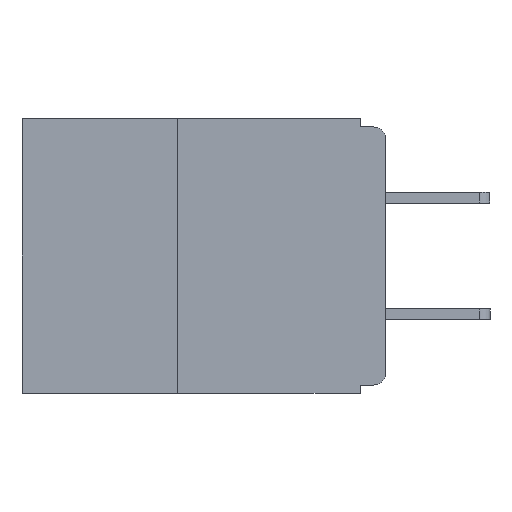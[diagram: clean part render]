
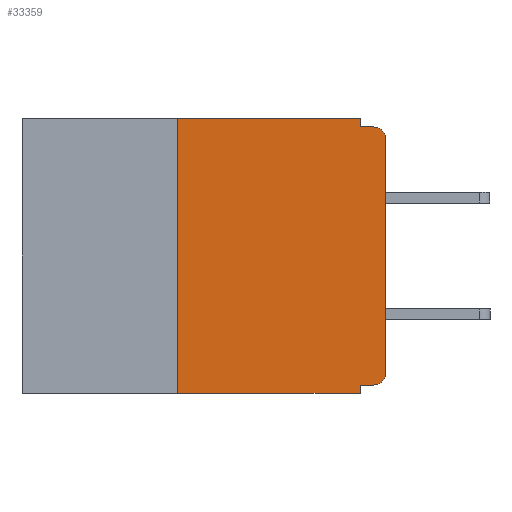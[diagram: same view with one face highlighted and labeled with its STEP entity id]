
A CAD part, left-side view. The second image highlights one B-rep face of the part: STEP entity #33359.
In plain terms, the highlighted planar face has unit normal (-1, 0, 0).
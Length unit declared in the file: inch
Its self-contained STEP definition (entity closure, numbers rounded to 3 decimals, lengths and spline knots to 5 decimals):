
#318 = DIRECTION ( 'NONE',  ( 0., 0., -1. ) ) ;
#726 = EDGE_CURVE ( 'NONE', #26985, #7900, #34645, .T. ) ;
#847 = CARTESIAN_POINT ( 'NONE',  ( 0., 0.031, 0. ) ) ;
#1365 = DIRECTION ( 'NONE',  ( 0., 0., -1. ) ) ;
#1405 = VECTOR ( 'NONE', #31967, 39.37008 ) ;
#1496 = EDGE_CURVE ( 'NONE', #7900, #27815, #26447, .T. ) ;
#2382 = EDGE_CURVE ( 'NONE', #5770, #13021, #21820, .T. ) ;
#3158 = CARTESIAN_POINT ( 'NONE',  ( 0., 0.437, 0. ) ) ;
#3741 = EDGE_CURVE ( 'NONE', #24078, #5770, #20894, .T. ) ;
#3787 = CARTESIAN_POINT ( 'NONE',  ( 0., 0., 0. ) ) ;
#3808 = ORIENTED_EDGE ( 'NONE', *, *, #24205, .T. ) ;
#3961 = AXIS2_PLACEMENT_3D ( 'NONE', #31239, #19602, #31909 ) ;
#4625 = ORIENTED_EDGE ( 'NONE', *, *, #31424, .F. ) ;
#4750 = DIRECTION ( 'NONE',  ( 0., 0., 1. ) ) ;
#5303 = CIRCLE ( 'NONE', #6736, 0.015 ) ;
#5507 = VERTEX_POINT ( 'NONE', #29978 ) ;
#5715 = CARTESIAN_POINT ( 'NONE',  ( 0., 0.015, -0.32 ) ) ;
#5770 = VERTEX_POINT ( 'NONE', #23873 ) ;
#6176 = EDGE_CURVE ( 'NONE', #10898, #5507, #14088, .T. ) ;
#6492 = EDGE_LOOP ( 'NONE', ( #9251, #15450, #22205, #30851, #4625, #8995, #25950, #33339, #33775, #3808 ) ) ;
#6518 = CARTESIAN_POINT ( 'NONE',  ( 0., 0.031, -0.33 ) ) ;
#6703 = DIRECTION ( 'NONE',  ( 0., 0., -1. ) ) ;
#6736 = AXIS2_PLACEMENT_3D ( 'NONE', #32849, #17003, #318 ) ;
#6877 = CARTESIAN_POINT ( 'NONE',  ( 0., 0.437, -0.33 ) ) ;
#7264 = EDGE_CURVE ( 'NONE', #29839, #27815, #22484, .T. ) ;
#7900 = VERTEX_POINT ( 'NONE', #11192 ) ;
#8308 = VECTOR ( 'NONE', #1365, 39.37008 ) ;
#8995 = ORIENTED_EDGE ( 'NONE', *, *, #6176, .F. ) ;
#9032 = EDGE_CURVE ( 'NONE', #15459, #29839, #22810, .T. ) ;
#9063 = VECTOR ( 'NONE', #17097, 39.37008 ) ;
#9251 = ORIENTED_EDGE ( 'NONE', *, *, #726, .T. ) ;
#9898 = LINE ( 'NONE', #3158, #9063 ) ;
#10804 = AXIS2_PLACEMENT_3D ( 'NONE', #30235, #14223, #32842 ) ;
#10898 = VERTEX_POINT ( 'NONE', #25825 ) ;
#11192 = CARTESIAN_POINT ( 'NONE',  ( 0., 0., -0.025 ) ) ;
#13021 = VERTEX_POINT ( 'NONE', #6518 ) ;
#13622 = VECTOR ( 'NONE', #25962, 39.37008 ) ;
#14088 = LINE ( 'NONE', #14890, #27540 ) ;
#14223 = DIRECTION ( 'NONE',  ( 1., 0., 0. ) ) ;
#14844 = DIRECTION ( 'NONE',  ( 0., 0., 1. ) ) ;
#14890 = CARTESIAN_POINT ( 'NONE',  ( 0., 0.25, -0.33 ) ) ;
#15450 = ORIENTED_EDGE ( 'NONE', *, *, #1496, .T. ) ;
#15459 = VERTEX_POINT ( 'NONE', #22122 ) ;
#15578 = CARTESIAN_POINT ( 'NONE',  ( 0., 0.031, -0.33 ) ) ;
#17003 = DIRECTION ( 'NONE',  ( -1., 0., 0. ) ) ;
#17097 = DIRECTION ( 'NONE',  ( 0., -1., 0. ) ) ;
#19602 = DIRECTION ( 'NONE',  ( -1., 0., 0. ) ) ;
#19837 = VECTOR ( 'NONE', #31117, 39.37008 ) ;
#20332 = EDGE_CURVE ( 'NONE', #10898, #13021, #22331, .T. ) ;
#20554 = CARTESIAN_POINT ( 'NONE',  ( 0., 0.031, -0.01 ) ) ;
#20894 = LINE ( 'NONE', #25460, #13622 ) ;
#21820 = LINE ( 'NONE', #15578, #34932 ) ;
#22122 = CARTESIAN_POINT ( 'NONE',  ( 0., 0.031, 0. ) ) ;
#22205 = ORIENTED_EDGE ( 'NONE', *, *, #7264, .F. ) ;
#22331 = LINE ( 'NONE', #6877, #19837 ) ;
#22484 = LINE ( 'NONE', #32838, #1405 ) ;
#22810 = LINE ( 'NONE', #847, #8308 ) ;
#23873 = CARTESIAN_POINT ( 'NONE',  ( 0., 0.031, -0.32 ) ) ;
#24078 = VERTEX_POINT ( 'NONE', #5715 ) ;
#24205 = EDGE_CURVE ( 'NONE', #24078, #26985, #5303, .T. ) ;
#25460 = CARTESIAN_POINT ( 'NONE',  ( 0., 0., -0.32 ) ) ;
#25825 = CARTESIAN_POINT ( 'NONE',  ( 0., 0.25, -0.33 ) ) ;
#25950 = ORIENTED_EDGE ( 'NONE', *, *, #20332, .T. ) ;
#25962 = DIRECTION ( 'NONE',  ( 0., 1., 0. ) ) ;
#26447 = CIRCLE ( 'NONE', #3961, 0.015 ) ;
#26985 = VERTEX_POINT ( 'NONE', #28382 ) ;
#27411 = CARTESIAN_POINT ( 'NONE',  ( 0., 0.015, -0.01 ) ) ;
#27540 = VECTOR ( 'NONE', #14844, 39.37008 ) ;
#27610 = PLANE ( 'NONE',  #10804 ) ;
#27735 = VECTOR ( 'NONE', #4750, 39.37008 ) ;
#27815 = VERTEX_POINT ( 'NONE', #27411 ) ;
#28382 = CARTESIAN_POINT ( 'NONE',  ( 0., 0., -0.305 ) ) ;
#29588 = FACE_OUTER_BOUND ( 'NONE', #6492, .T. ) ;
#29839 = VERTEX_POINT ( 'NONE', #20554 ) ;
#29978 = CARTESIAN_POINT ( 'NONE',  ( 0., 0.25, 0. ) ) ;
#30235 = CARTESIAN_POINT ( 'NONE',  ( 0., 0.437, 0. ) ) ;
#30851 = ORIENTED_EDGE ( 'NONE', *, *, #9032, .F. ) ;
#31117 = DIRECTION ( 'NONE',  ( 0., -1., 0. ) ) ;
#31239 = CARTESIAN_POINT ( 'NONE',  ( 0., 0.015, -0.025 ) ) ;
#31424 = EDGE_CURVE ( 'NONE', #5507, #15459, #9898, .T. ) ;
#31909 = DIRECTION ( 'NONE',  ( 0., 0., -1. ) ) ;
#31967 = DIRECTION ( 'NONE',  ( 0., -1., 0. ) ) ;
#32838 = CARTESIAN_POINT ( 'NONE',  ( 0., 0., -0.01 ) ) ;
#32842 = DIRECTION ( 'NONE',  ( 0., 0., -1. ) ) ;
#32849 = CARTESIAN_POINT ( 'NONE',  ( 0., 0.015, -0.305 ) ) ;
#33339 = ORIENTED_EDGE ( 'NONE', *, *, #2382, .F. ) ;
#33359 = ADVANCED_FACE ( 'NONE', ( #29588 ), #27610, .F. ) ;
#33775 = ORIENTED_EDGE ( 'NONE', *, *, #3741, .F. ) ;
#34645 = LINE ( 'NONE', #3787, #27735 ) ;
#34932 = VECTOR ( 'NONE', #6703, 39.37008 ) ;
